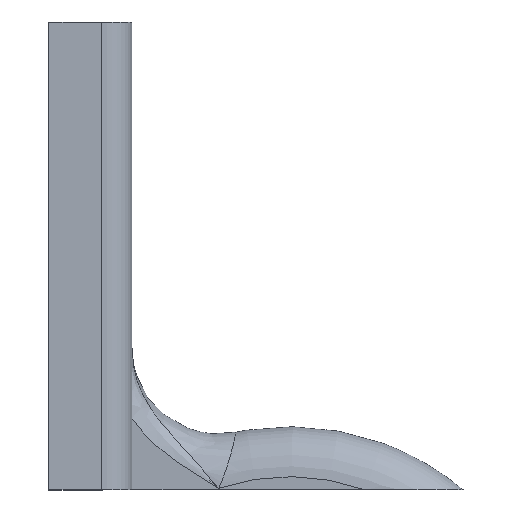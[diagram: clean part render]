
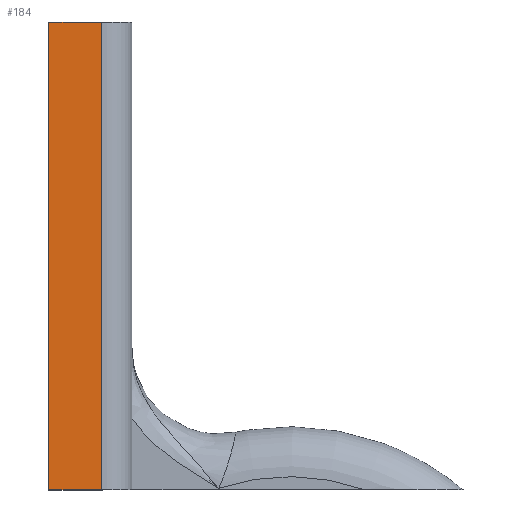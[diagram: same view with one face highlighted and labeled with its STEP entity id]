
A CAD part, left-side view. The second image highlights one B-rep face of the part: STEP entity #184.
In plain terms, the highlighted planar face has unit normal (-1, 0, 0).
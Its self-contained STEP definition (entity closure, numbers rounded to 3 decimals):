
#184 = ADVANCED_FACE ( 'NONE', ( #646 ), #643, .F. ) ;
#281 = VECTOR ( 'NONE', #1255, 1000. ) ;
#284 = VECTOR ( 'NONE', #1260, 1000. ) ;
#286 = LINE ( 'NONE', #1467, #281 ) ;
#287 = VECTOR ( 'NONE', #1248, 1000. ) ;
#290 = LINE ( 'NONE', #1241, #284 ) ;
#309 = LINE ( 'NONE', #1383, #287 ) ;
#314 = VECTOR ( 'NONE', #430, 1000. ) ;
#334 = LINE ( 'NONE', #361, #314 ) ;
#361 = CARTESIAN_POINT ( 'NONE',  ( -175.989, 21.06, -35.859 ) ) ;
#430 = DIRECTION ( 'NONE',  ( 0., 1., 0. ) ) ;
#536 = CARTESIAN_POINT ( 'NONE',  ( -175.989, 21.06, -35.859 ) ) ;
#582 = DIRECTION ( 'NONE',  ( 1., 0., 0. ) ) ;
#643 = PLANE ( 'NONE',  #1824 ) ;
#646 = FACE_OUTER_BOUND ( 'NONE', #900, .T. ) ;
#680 = DIRECTION ( 'NONE',  ( 0., 0., -1. ) ) ;
#794 = CARTESIAN_POINT ( 'NONE',  ( -175.989, 21.06, 72.14 ) ) ;
#800 = CARTESIAN_POINT ( 'NONE',  ( -175.989, 33.179, -35.859 ) ) ;
#818 = CARTESIAN_POINT ( 'NONE',  ( -175.989, 33.179, 72.14 ) ) ;
#853 = VERTEX_POINT ( 'NONE', #818 ) ;
#867 = VERTEX_POINT ( 'NONE', #800 ) ;
#871 = VERTEX_POINT ( 'NONE', #794 ) ;
#888 = VERTEX_POINT ( 'NONE', #536 ) ;
#900 = EDGE_LOOP ( 'NONE', ( #1712, #1749, #1773, #1783 ) ) ;
#1065 = CARTESIAN_POINT ( 'NONE',  ( -175.989, 21.06, -281.105 ) ) ;
#1241 = CARTESIAN_POINT ( 'NONE',  ( -175.989, 48.821, 72.14 ) ) ;
#1248 = DIRECTION ( 'NONE',  ( 0., 0., -1. ) ) ;
#1255 = DIRECTION ( 'NONE',  ( 0., 0., 1. ) ) ;
#1260 = DIRECTION ( 'NONE',  ( 0., -1., 0. ) ) ;
#1383 = CARTESIAN_POINT ( 'NONE',  ( -175.989, 21.06, -281.105 ) ) ;
#1467 = CARTESIAN_POINT ( 'NONE',  ( -175.989, 33.179, -302.609 ) ) ;
#1712 = ORIENTED_EDGE ( 'NONE', *, *, #1995, .F. ) ;
#1749 = ORIENTED_EDGE ( 'NONE', *, *, #2025, .F. ) ;
#1773 = ORIENTED_EDGE ( 'NONE', *, *, #2029, .F. ) ;
#1783 = ORIENTED_EDGE ( 'NONE', *, *, #2031, .F. ) ;
#1824 = AXIS2_PLACEMENT_3D ( 'NONE', #1065, #582, #680 ) ;
#1995 = EDGE_CURVE ( 'NONE', #888, #867, #334, .T. ) ;
#2025 = EDGE_CURVE ( 'NONE', #871, #888, #309, .T. ) ;
#2029 = EDGE_CURVE ( 'NONE', #853, #871, #290, .T. ) ;
#2031 = EDGE_CURVE ( 'NONE', #867, #853, #286, .T. ) ;
